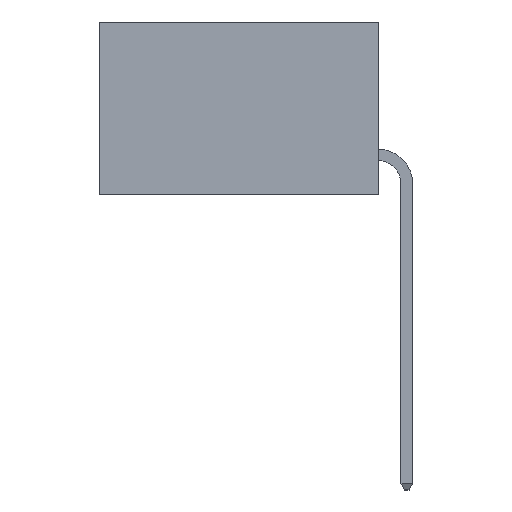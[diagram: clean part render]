
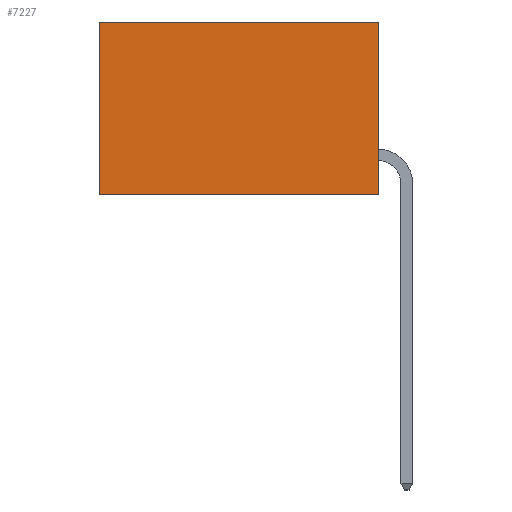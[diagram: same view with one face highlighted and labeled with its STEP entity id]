
A CAD part, left-side view. The second image highlights one B-rep face of the part: STEP entity #7227.
In plain terms, the highlighted planar face has unit normal (-1, 0, 0).
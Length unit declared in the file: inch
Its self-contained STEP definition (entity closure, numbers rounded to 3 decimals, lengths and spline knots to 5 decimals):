
#4 = EDGE_CURVE ( 'NONE', #240, #15799, #6539, .T. ) ;
#240 = VERTEX_POINT ( 'NONE', #5112 ) ;
#400 = VERTEX_POINT ( 'NONE', #15762 ) ;
#667 = ORIENTED_EDGE ( 'NONE', *, *, #6752, .T. ) ;
#823 = EDGE_LOOP ( 'NONE', ( #11297, #14013, #10975, #667 ) ) ;
#1557 = DIRECTION ( 'NONE',  ( 0., 0., -1. ) ) ;
#2894 = VECTOR ( 'NONE', #14653, 39.37008 ) ;
#3062 = VECTOR ( 'NONE', #1557, 39.37008 ) ;
#3297 = VECTOR ( 'NONE', #10460, 39.37008 ) ;
#3313 = LINE ( 'NONE', #7357, #2894 ) ;
#4088 = CARTESIAN_POINT ( 'NONE',  ( 0.2615, 0., -0.37 ) ) ;
#4115 = DIRECTION ( 'NONE',  ( 0., 1., 0. ) ) ;
#4498 = CARTESIAN_POINT ( 'NONE',  ( 0.2615, 0., -0.37 ) ) ;
#4538 = EDGE_CURVE ( 'NONE', #15799, #7166, #8653, .T. ) ;
#4798 = VECTOR ( 'NONE', #4115, 39.37008 ) ;
#5112 = CARTESIAN_POINT ( 'NONE',  ( 0.2615, 0., 0. ) ) ;
#5801 = DIRECTION ( 'NONE',  ( 0., 0., -1. ) ) ;
#6539 = LINE ( 'NONE', #9406, #3062 ) ;
#6752 = EDGE_CURVE ( 'NONE', #240, #400, #3313, .T. ) ;
#7166 = VERTEX_POINT ( 'NONE', #15464 ) ;
#7227 = ADVANCED_FACE ( 'NONE', ( #15360 ), #12003, .F. ) ;
#7357 = CARTESIAN_POINT ( 'NONE',  ( 0.2615, 0., 0. ) ) ;
#8653 = LINE ( 'NONE', #4088, #4798 ) ;
#9274 = CARTESIAN_POINT ( 'NONE',  ( 0.2615, 0.6, -0.37 ) ) ;
#9406 = CARTESIAN_POINT ( 'NONE',  ( 0.2615, 0., -0.37 ) ) ;
#10460 = DIRECTION ( 'NONE',  ( 0., 0., -1. ) ) ;
#10853 = LINE ( 'NONE', #9274, #3297 ) ;
#10975 = ORIENTED_EDGE ( 'NONE', *, *, #4, .F. ) ;
#11297 = ORIENTED_EDGE ( 'NONE', *, *, #15024, .T. ) ;
#12003 = PLANE ( 'NONE',  #13522 ) ;
#13248 = DIRECTION ( 'NONE',  ( 1., 0., 0. ) ) ;
#13522 = AXIS2_PLACEMENT_3D ( 'NONE', #4498, #13248, #5801 ) ;
#14013 = ORIENTED_EDGE ( 'NONE', *, *, #4538, .F. ) ;
#14653 = DIRECTION ( 'NONE',  ( 0., 1., 0. ) ) ;
#15024 = EDGE_CURVE ( 'NONE', #400, #7166, #10853, .T. ) ;
#15360 = FACE_OUTER_BOUND ( 'NONE', #823, .T. ) ;
#15464 = CARTESIAN_POINT ( 'NONE',  ( 0.2615, 0.6, -0.37 ) ) ;
#15572 = CARTESIAN_POINT ( 'NONE',  ( 0.2615, 0., -0.37 ) ) ;
#15762 = CARTESIAN_POINT ( 'NONE',  ( 0.2615, 0.6, 0. ) ) ;
#15799 = VERTEX_POINT ( 'NONE', #15572 ) ;
